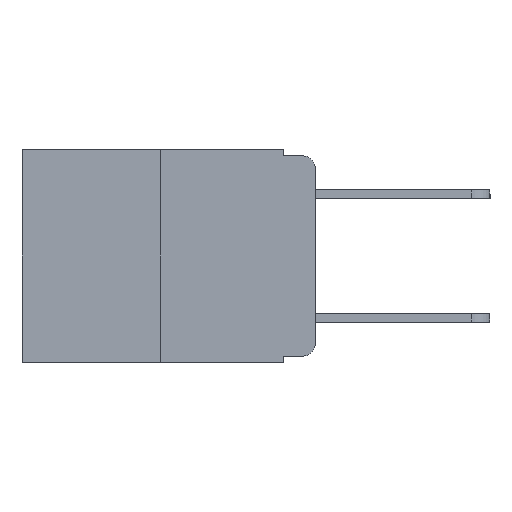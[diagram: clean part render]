
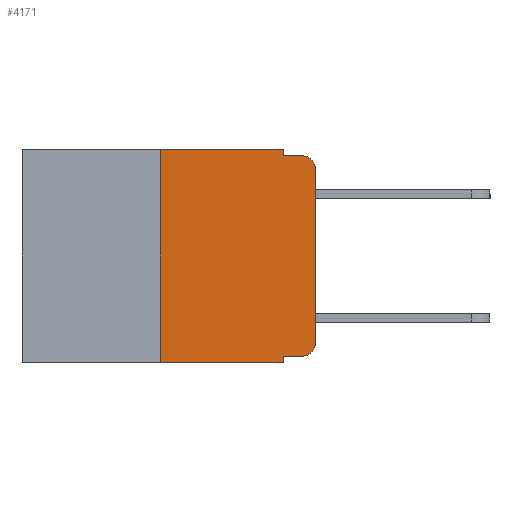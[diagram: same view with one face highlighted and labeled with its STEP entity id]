
A CAD part, left-side view. The second image highlights one B-rep face of the part: STEP entity #4171.
In plain terms, the highlighted planar face has unit normal (-1, 0, 0).
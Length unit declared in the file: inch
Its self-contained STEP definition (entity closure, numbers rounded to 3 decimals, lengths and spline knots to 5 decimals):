
#72 = CIRCLE ( 'NONE', #2317, 0.02 ) ;
#130 = VECTOR ( 'NONE', #10527, 39.37008 ) ;
#228 = CARTESIAN_POINT ( 'NONE',  ( 0., 0., 0. ) ) ;
#311 = VERTEX_POINT ( 'NONE', #7953 ) ;
#491 = EDGE_CURVE ( 'NONE', #702, #3568, #9982, .T. ) ;
#614 = LINE ( 'NONE', #9095, #4523 ) ;
#702 = VERTEX_POINT ( 'NONE', #4669 ) ;
#939 = VERTEX_POINT ( 'NONE', #8750 ) ;
#1241 = EDGE_CURVE ( 'NONE', #4298, #2699, #4368, .T. ) ;
#1294 = EDGE_CURVE ( 'NONE', #2699, #311, #8062, .T. ) ;
#1327 = EDGE_CURVE ( 'NONE', #1508, #311, #7641, .T. ) ;
#1342 = EDGE_CURVE ( 'NONE', #5259, #1508, #9751, .T. ) ;
#1362 = EDGE_CURVE ( 'NONE', #702, #9612, #5137, .T. ) ;
#1381 = EDGE_CURVE ( 'NONE', #939, #3568, #2376, .T. ) ;
#1400 = EDGE_CURVE ( 'NONE', #939, #4451, #614, .T. ) ;
#1403 = EDGE_CURVE ( 'NONE', #4451, #4298, #72, .T. ) ;
#1455 = ORIENTED_EDGE ( 'NONE', *, *, #1327, .F. ) ;
#1457 = CARTESIAN_POINT ( 'NONE',  ( 0., 0.473, 0. ) ) ;
#1463 = PLANE ( 'NONE',  #10264 ) ;
#1479 = ORIENTED_EDGE ( 'NONE', *, *, #6538, .F. ) ;
#1508 = VERTEX_POINT ( 'NONE', #7605 ) ;
#1736 = ORIENTED_EDGE ( 'NONE', *, *, #1362, .F. ) ;
#1772 = AXIS2_PLACEMENT_3D ( 'NONE', #7663, #7656, #6984 ) ;
#1933 = EDGE_LOOP ( 'NONE', ( #4967, #3231, #1455, #2503, #1479, #1736, #3855, #3579, #6373, #6118 ) ) ;
#2317 = AXIS2_PLACEMENT_3D ( 'NONE', #7253, #7240, #7230 ) ;
#2376 = LINE ( 'NONE', #9129, #8911 ) ;
#2429 = LINE ( 'NONE', #9828, #130 ) ;
#2503 = ORIENTED_EDGE ( 'NONE', *, *, #1342, .F. ) ;
#2630 = VECTOR ( 'NONE', #4589, 39.37008 ) ;
#2642 = CARTESIAN_POINT ( 'NONE',  ( 0., 0.02, -0.333 ) ) ;
#2699 = VERTEX_POINT ( 'NONE', #5470 ) ;
#3231 = ORIENTED_EDGE ( 'NONE', *, *, #1294, .T. ) ;
#3568 = VERTEX_POINT ( 'NONE', #4234 ) ;
#3579 = ORIENTED_EDGE ( 'NONE', *, *, #1381, .F. ) ;
#3855 = ORIENTED_EDGE ( 'NONE', *, *, #491, .T. ) ;
#4171 = ADVANCED_FACE ( 'NONE', ( #7019 ), #1463, .F. ) ;
#4234 = CARTESIAN_POINT ( 'NONE',  ( 0., 0.051, -0.343 ) ) ;
#4298 = VERTEX_POINT ( 'NONE', #5134 ) ;
#4368 = LINE ( 'NONE', #228, #8568 ) ;
#4451 = VERTEX_POINT ( 'NONE', #2642 ) ;
#4523 = VECTOR ( 'NONE', #9221, 39.37008 ) ;
#4527 = DIRECTION ( 'NONE',  ( 0., 0., -1. ) ) ;
#4589 = DIRECTION ( 'NONE',  ( 0., 0., 1. ) ) ;
#4669 = CARTESIAN_POINT ( 'NONE',  ( 0., 0.25, -0.343 ) ) ;
#4967 = ORIENTED_EDGE ( 'NONE', *, *, #1241, .T. ) ;
#5134 = CARTESIAN_POINT ( 'NONE',  ( 0., 0., -0.313 ) ) ;
#5137 = LINE ( 'NONE', #9329, #2630 ) ;
#5259 = VERTEX_POINT ( 'NONE', #6665 ) ;
#5422 = VECTOR ( 'NONE', #8256, 39.37008 ) ;
#5470 = CARTESIAN_POINT ( 'NONE',  ( 0., 0., -0.03 ) ) ;
#5856 = DIRECTION ( 'NONE',  ( 1., 0., 0. ) ) ;
#6118 = ORIENTED_EDGE ( 'NONE', *, *, #1403, .T. ) ;
#6373 = ORIENTED_EDGE ( 'NONE', *, *, #1400, .T. ) ;
#6538 = EDGE_CURVE ( 'NONE', #9612, #5259, #2429, .T. ) ;
#6665 = CARTESIAN_POINT ( 'NONE',  ( 0., 0.051, 0. ) ) ;
#6984 = DIRECTION ( 'NONE',  ( 0., 0., -1. ) ) ;
#7019 = FACE_OUTER_BOUND ( 'NONE', #1933, .T. ) ;
#7230 = DIRECTION ( 'NONE',  ( 0., 0., -1. ) ) ;
#7240 = DIRECTION ( 'NONE',  ( -1., 0., 0. ) ) ;
#7253 = CARTESIAN_POINT ( 'NONE',  ( 0., 0.02, -0.313 ) ) ;
#7390 = DIRECTION ( 'NONE',  ( 0., 0., -1. ) ) ;
#7605 = CARTESIAN_POINT ( 'NONE',  ( 0., 0.051, -0.01 ) ) ;
#7641 = LINE ( 'NONE', #9501, #5422 ) ;
#7656 = DIRECTION ( 'NONE',  ( -1., 0., 0. ) ) ;
#7663 = CARTESIAN_POINT ( 'NONE',  ( 0., 0.02, -0.03 ) ) ;
#7953 = CARTESIAN_POINT ( 'NONE',  ( 0., 0.02, -0.01 ) ) ;
#8062 = CIRCLE ( 'NONE', #1772, 0.02 ) ;
#8256 = DIRECTION ( 'NONE',  ( 0., -1., 0. ) ) ;
#8568 = VECTOR ( 'NONE', #9682, 39.37008 ) ;
#8750 = CARTESIAN_POINT ( 'NONE',  ( 0., 0.051, -0.333 ) ) ;
#8911 = VECTOR ( 'NONE', #9283, 39.37008 ) ;
#9095 = CARTESIAN_POINT ( 'NONE',  ( 0., 0.051, -0.333 ) ) ;
#9129 = CARTESIAN_POINT ( 'NONE',  ( 0., 0.051, 0. ) ) ;
#9221 = DIRECTION ( 'NONE',  ( 0., -1., 0. ) ) ;
#9283 = DIRECTION ( 'NONE',  ( 0., 0., -1. ) ) ;
#9285 = CARTESIAN_POINT ( 'NONE',  ( 0., 0.051, 0. ) ) ;
#9329 = CARTESIAN_POINT ( 'NONE',  ( 0., 0.25, 0. ) ) ;
#9501 = CARTESIAN_POINT ( 'NONE',  ( 0., 0.051, -0.01 ) ) ;
#9557 = VECTOR ( 'NONE', #7390, 39.37008 ) ;
#9612 = VERTEX_POINT ( 'NONE', #10167 ) ;
#9682 = DIRECTION ( 'NONE',  ( 0., 0., 1. ) ) ;
#9751 = LINE ( 'NONE', #9285, #9557 ) ;
#9763 = VECTOR ( 'NONE', #9777, 39.37008 ) ;
#9777 = DIRECTION ( 'NONE',  ( 0., -1., 0. ) ) ;
#9819 = CARTESIAN_POINT ( 'NONE',  ( 0., 0.473, -0.343 ) ) ;
#9828 = CARTESIAN_POINT ( 'NONE',  ( 0., 0.473, 0. ) ) ;
#9982 = LINE ( 'NONE', #9819, #9763 ) ;
#10167 = CARTESIAN_POINT ( 'NONE',  ( 0., 0.25, 0. ) ) ;
#10264 = AXIS2_PLACEMENT_3D ( 'NONE', #1457, #5856, #4527 ) ;
#10527 = DIRECTION ( 'NONE',  ( 0., -1., 0. ) ) ;
